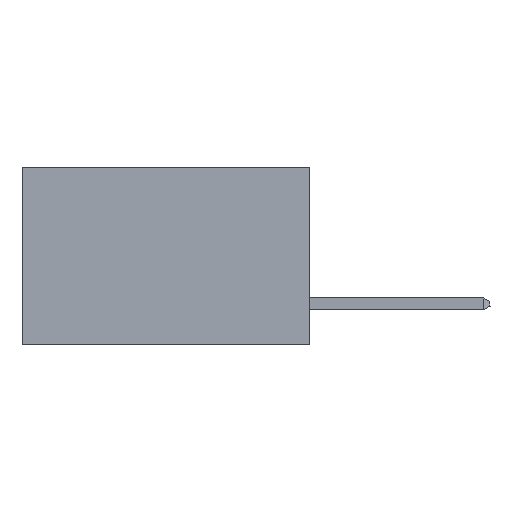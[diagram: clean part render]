
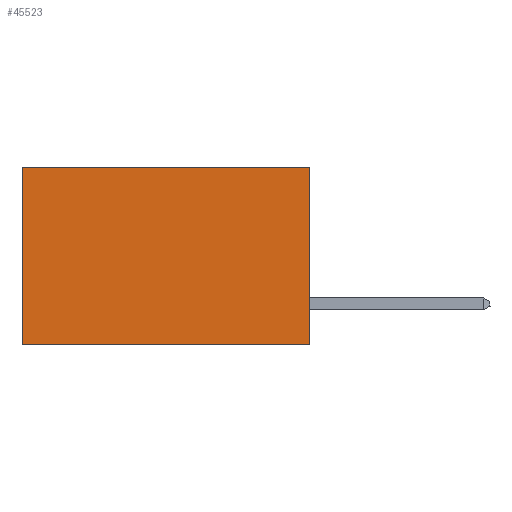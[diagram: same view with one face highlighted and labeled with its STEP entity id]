
A CAD part, left-side view. The second image highlights one B-rep face of the part: STEP entity #45523.
In plain terms, the highlighted planar face has unit normal (-1, 0, 0).
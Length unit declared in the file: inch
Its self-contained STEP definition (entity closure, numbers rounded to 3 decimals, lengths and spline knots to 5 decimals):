
#4650 = AXIS2_PLACEMENT_3D ( 'NONE', #22675, #8526, #26242 ) ;
#5201 = CARTESIAN_POINT ( 'NONE',  ( 0.2875, 0., -0.37 ) ) ;
#8008 = CARTESIAN_POINT ( 'NONE',  ( 0.2875, 0.6, -0.37 ) ) ;
#8526 = DIRECTION ( 'NONE',  ( 1., 0., 0. ) ) ;
#9237 = EDGE_CURVE ( 'NONE', #29611, #17654, #33584, .T. ) ;
#10700 = VERTEX_POINT ( 'NONE', #37592 ) ;
#13857 = ORIENTED_EDGE ( 'NONE', *, *, #15273, .F. ) ;
#14417 = CARTESIAN_POINT ( 'NONE',  ( 0.2875, 0., -0.37 ) ) ;
#15273 = EDGE_CURVE ( 'NONE', #45184, #29611, #44162, .T. ) ;
#15853 = ORIENTED_EDGE ( 'NONE', *, *, #33200, .T. ) ;
#15939 = VECTOR ( 'NONE', #37765, 39.37008 ) ;
#17654 = VERTEX_POINT ( 'NONE', #8008 ) ;
#19632 = VECTOR ( 'NONE', #22809, 39.37008 ) ;
#21329 = ORIENTED_EDGE ( 'NONE', *, *, #9237, .F. ) ;
#21842 = LINE ( 'NONE', #31718, #19632 ) ;
#22675 = CARTESIAN_POINT ( 'NONE',  ( 0.2875, 0., 0. ) ) ;
#22774 = DIRECTION ( 'NONE',  ( 0., 1., 0. ) ) ;
#22809 = DIRECTION ( 'NONE',  ( 0., 1., 0. ) ) ;
#23341 = CARTESIAN_POINT ( 'NONE',  ( 0.2875, 0., 0. ) ) ;
#24252 = CARTESIAN_POINT ( 'NONE',  ( 0.2875, 0.6, 0. ) ) ;
#26242 = DIRECTION ( 'NONE',  ( 0., 0., -1. ) ) ;
#29100 = VECTOR ( 'NONE', #22774, 39.37008 ) ;
#29611 = VERTEX_POINT ( 'NONE', #14417 ) ;
#29830 = PLANE ( 'NONE',  #4650 ) ;
#31718 = CARTESIAN_POINT ( 'NONE',  ( 0.2875, 0., 0. ) ) ;
#31738 = EDGE_LOOP ( 'NONE', ( #33702, #21329, #13857, #15853 ) ) ;
#33200 = EDGE_CURVE ( 'NONE', #45184, #10700, #21842, .T. ) ;
#33584 = LINE ( 'NONE', #5201, #29100 ) ;
#33702 = ORIENTED_EDGE ( 'NONE', *, *, #41675, .T. ) ;
#33741 = DIRECTION ( 'NONE',  ( 0., 0., -1. ) ) ;
#34722 = VECTOR ( 'NONE', #33741, 39.37008 ) ;
#37148 = CARTESIAN_POINT ( 'NONE',  ( 0.2875, 0., 0. ) ) ;
#37592 = CARTESIAN_POINT ( 'NONE',  ( 0.2875, 0.6, 0. ) ) ;
#37765 = DIRECTION ( 'NONE',  ( 0., 0., -1. ) ) ;
#40108 = FACE_OUTER_BOUND ( 'NONE', #31738, .T. ) ;
#41675 = EDGE_CURVE ( 'NONE', #10700, #17654, #44378, .T. ) ;
#44162 = LINE ( 'NONE', #37148, #34722 ) ;
#44378 = LINE ( 'NONE', #24252, #15939 ) ;
#45184 = VERTEX_POINT ( 'NONE', #23341 ) ;
#45523 = ADVANCED_FACE ( 'NONE', ( #40108 ), #29830, .F. ) ;
